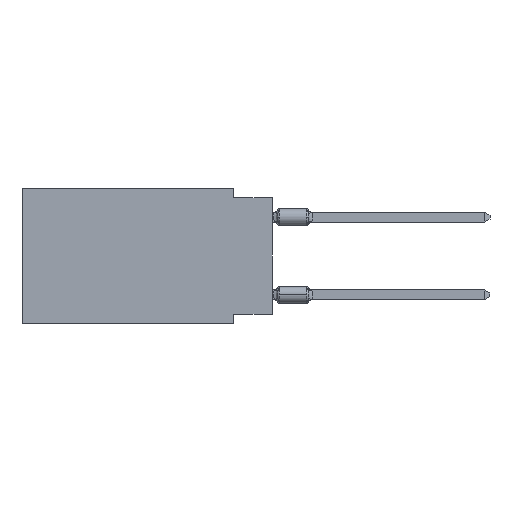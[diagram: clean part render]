
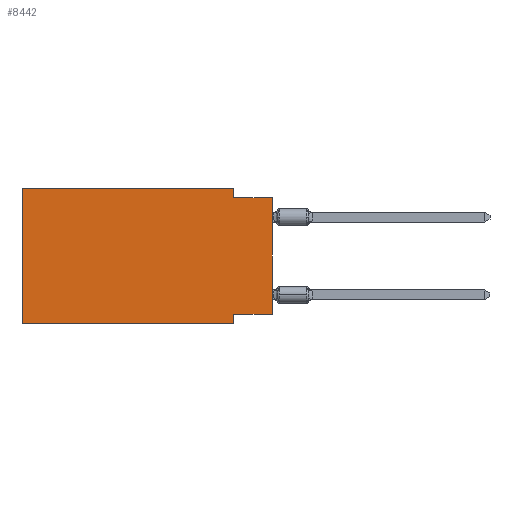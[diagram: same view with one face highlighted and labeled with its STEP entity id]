
A CAD part, left-side view. The second image highlights one B-rep face of the part: STEP entity #8442.
In plain terms, the highlighted planar face has unit normal (-1, 0, 0).
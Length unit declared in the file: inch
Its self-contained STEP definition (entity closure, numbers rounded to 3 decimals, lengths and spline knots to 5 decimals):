
#45 = DIRECTION ( 'NONE',  ( 0., 0., 1. ) ) ;
#114 = CARTESIAN_POINT ( 'NONE',  ( 0., 0.645, 0. ) ) ;
#1058 = VECTOR ( 'NONE', #45, 39.37008 ) ;
#1090 = LINE ( 'NONE', #9500, #1058 ) ;
#1291 = ORIENTED_EDGE ( 'NONE', *, *, #13104, .T. ) ;
#1398 = LINE ( 'NONE', #12981, #12216 ) ;
#1985 = CARTESIAN_POINT ( 'NONE',  ( 0., 0., -0.025 ) ) ;
#2488 = VERTEX_POINT ( 'NONE', #7038 ) ;
#2892 = LINE ( 'NONE', #11370, #3456 ) ;
#3055 = EDGE_CURVE ( 'NONE', #10751, #5345, #9359, .T. ) ;
#3275 = LINE ( 'NONE', #1985, #3648 ) ;
#3293 = DIRECTION ( 'NONE',  ( 0., -1., 0. ) ) ;
#3456 = VECTOR ( 'NONE', #7080, 39.37008 ) ;
#3550 = EDGE_CURVE ( 'NONE', #2488, #11689, #3275, .T. ) ;
#3614 = CARTESIAN_POINT ( 'NONE',  ( 0., 0.1, 0. ) ) ;
#3648 = VECTOR ( 'NONE', #6171, 39.37008 ) ;
#3823 = DIRECTION ( 'NONE',  ( 0., 0., -1. ) ) ;
#4046 = CARTESIAN_POINT ( 'NONE',  ( 0., 0.645, -0.35 ) ) ;
#4498 = ORIENTED_EDGE ( 'NONE', *, *, #11726, .F. ) ;
#4582 = VECTOR ( 'NONE', #10674, 39.37008 ) ;
#4818 = ORIENTED_EDGE ( 'NONE', *, *, #3055, .F. ) ;
#4852 = CARTESIAN_POINT ( 'NONE',  ( 0., 0.645, 0. ) ) ;
#5146 = VECTOR ( 'NONE', #11215, 39.37008 ) ;
#5303 = CARTESIAN_POINT ( 'NONE',  ( 0., 0.1, -0.325 ) ) ;
#5345 = VERTEX_POINT ( 'NONE', #3614 ) ;
#5398 = EDGE_CURVE ( 'NONE', #6890, #10231, #8992, .T. ) ;
#5705 = VECTOR ( 'NONE', #11498, 39.37008 ) ;
#6171 = DIRECTION ( 'NONE',  ( 0., -1., 0. ) ) ;
#6730 = EDGE_CURVE ( 'NONE', #5345, #2488, #1398, .T. ) ;
#6841 = ORIENTED_EDGE ( 'NONE', *, *, #10454, .T. ) ;
#6890 = VERTEX_POINT ( 'NONE', #12085 ) ;
#6899 = CARTESIAN_POINT ( 'NONE',  ( 0., 0.1, -0.35 ) ) ;
#6963 = VECTOR ( 'NONE', #3293, 39.37008 ) ;
#7031 = ORIENTED_EDGE ( 'NONE', *, *, #3550, .F. ) ;
#7038 = CARTESIAN_POINT ( 'NONE',  ( 0., 0.1, -0.025 ) ) ;
#7060 = VERTEX_POINT ( 'NONE', #12409 ) ;
#7080 = DIRECTION ( 'NONE',  ( 0., 0., 1. ) ) ;
#7134 = LINE ( 'NONE', #4046, #5705 ) ;
#7811 = CARTESIAN_POINT ( 'NONE',  ( 0., 0., -0.325 ) ) ;
#8442 = ADVANCED_FACE ( 'NONE', ( #13269 ), #10225, .F. ) ;
#8566 = DIRECTION ( 'NONE',  ( 0., 0., -1. ) ) ;
#8592 = CARTESIAN_POINT ( 'NONE',  ( 0., 0.1, -0.35 ) ) ;
#8992 = LINE ( 'NONE', #7811, #5146 ) ;
#9143 = CARTESIAN_POINT ( 'NONE',  ( 0., 0.645, 0. ) ) ;
#9359 = LINE ( 'NONE', #114, #6963 ) ;
#9500 = CARTESIAN_POINT ( 'NONE',  ( 0., 0.645, 0. ) ) ;
#10225 = PLANE ( 'NONE',  #13539 ) ;
#10231 = VERTEX_POINT ( 'NONE', #5303 ) ;
#10454 = EDGE_CURVE ( 'NONE', #6890, #11689, #2892, .T. ) ;
#10674 = DIRECTION ( 'NONE',  ( 0., 0., -1. ) ) ;
#10751 = VERTEX_POINT ( 'NONE', #9143 ) ;
#10932 = ORIENTED_EDGE ( 'NONE', *, *, #5398, .F. ) ;
#11215 = DIRECTION ( 'NONE',  ( 0., 1., 0. ) ) ;
#11370 = CARTESIAN_POINT ( 'NONE',  ( 0., 0., 0. ) ) ;
#11498 = DIRECTION ( 'NONE',  ( 0., -1., 0. ) ) ;
#11689 = VERTEX_POINT ( 'NONE', #13573 ) ;
#11698 = LINE ( 'NONE', #8592, #4582 ) ;
#11726 = EDGE_CURVE ( 'NONE', #10231, #12161, #11698, .T. ) ;
#11762 = EDGE_CURVE ( 'NONE', #7060, #10751, #1090, .T. ) ;
#12085 = CARTESIAN_POINT ( 'NONE',  ( 0., 0., -0.325 ) ) ;
#12161 = VERTEX_POINT ( 'NONE', #6899 ) ;
#12216 = VECTOR ( 'NONE', #8566, 39.37008 ) ;
#12285 = ORIENTED_EDGE ( 'NONE', *, *, #11762, .F. ) ;
#12286 = DIRECTION ( 'NONE',  ( 1., 0., 0. ) ) ;
#12409 = CARTESIAN_POINT ( 'NONE',  ( 0., 0.645, -0.35 ) ) ;
#12615 = EDGE_LOOP ( 'NONE', ( #6841, #7031, #12982, #4818, #12285, #1291, #4498, #10932 ) ) ;
#12981 = CARTESIAN_POINT ( 'NONE',  ( 0., 0.1, 0. ) ) ;
#12982 = ORIENTED_EDGE ( 'NONE', *, *, #6730, .F. ) ;
#13104 = EDGE_CURVE ( 'NONE', #7060, #12161, #7134, .T. ) ;
#13269 = FACE_OUTER_BOUND ( 'NONE', #12615, .T. ) ;
#13539 = AXIS2_PLACEMENT_3D ( 'NONE', #4852, #12286, #3823 ) ;
#13573 = CARTESIAN_POINT ( 'NONE',  ( 0., 0., -0.025 ) ) ;
